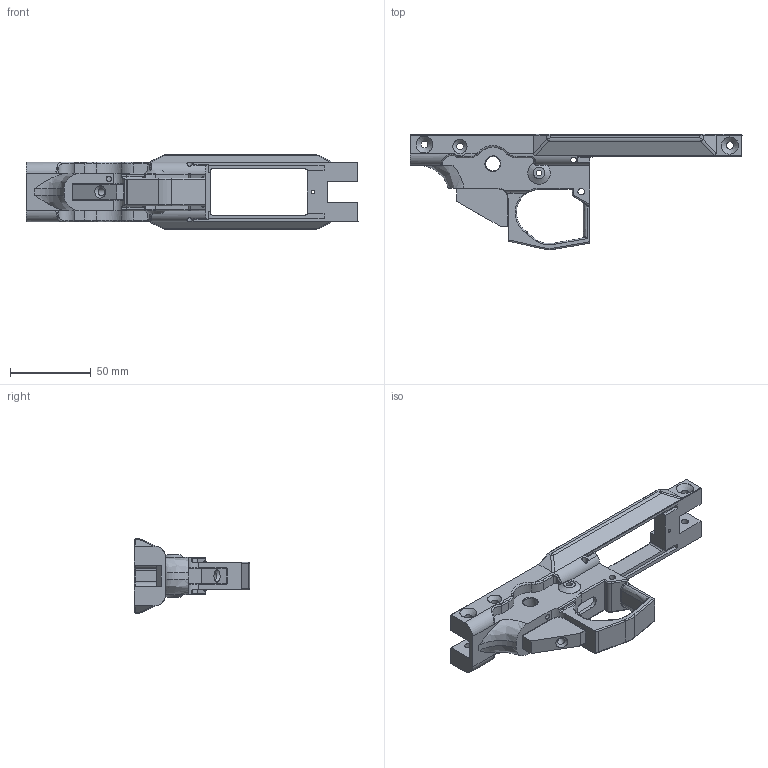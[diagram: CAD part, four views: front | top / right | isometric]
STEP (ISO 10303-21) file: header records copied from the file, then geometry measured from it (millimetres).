
FILE_DESCRIPTION (( 'STEP AP203' ), '1' );
FILE_NAME ('MOD9_lower_receiver.STEP', '2020-06-10T04:59:30', ( '' ), ( '' ), 'SwSTEP 2.0', 'SolidWorks 2016', '' );
FILE_SCHEMA (( 'CONFIG_CONTROL_DESIGN' ));
Length unit declared in the file: millimetre
Products named in the file (1): MOD9_lower_receiver
Bounding box: 205.55 x 71.26 x 46.13 mm (x, y, z)
Volume: 101147.8 mm3; surface area: 39394.5 mm2
Topology: 1 solids, 1 shells, 337 faces, 912 edges, 560 vertices
Faces by surface type: plane 124, cylinder 118, bspline 67, cone 28
Full cylindrical faces by diameter (mm): 2 x1, 3.175 x1, 3.469 x4, 4 x1, 4.175 x2, 4.4 x2, 4.6 x2, 4.605 x1, 9.025 x2
Entity records: 17710 total; most frequent: CARTESIAN_POINT 10204, ORIENTED_EDGE 1692, DIRECTION 1260, EDGE_CURVE 846, VERTEX_POINT 534, LINE 432, VECTOR 432, AXIS2_PLACEMENT_3D 414
